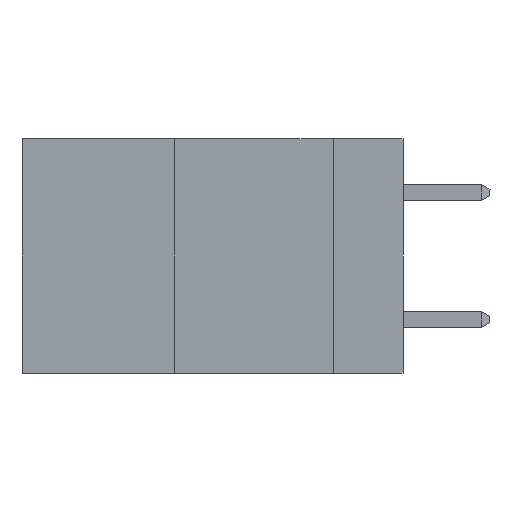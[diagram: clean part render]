
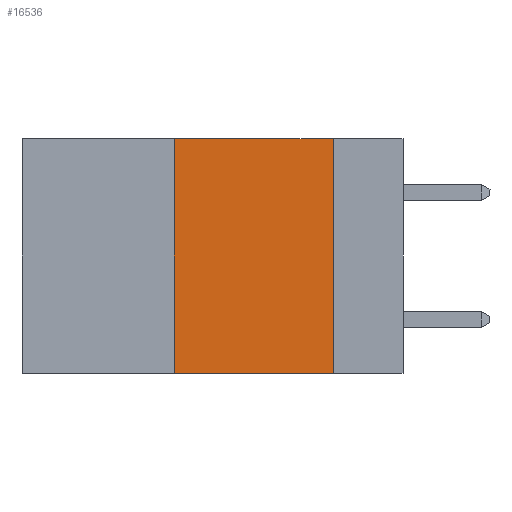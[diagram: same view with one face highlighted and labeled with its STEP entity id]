
A CAD part, left-side view. The second image highlights one B-rep face of the part: STEP entity #16536.
In plain terms, the highlighted planar face has unit normal (-1, 0, 0).
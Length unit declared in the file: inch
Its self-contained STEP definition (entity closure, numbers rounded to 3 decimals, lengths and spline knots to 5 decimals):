
#188 = EDGE_CURVE ( 'NONE', #3211, #1576, #2020, .T. ) ;
#1083 = DIRECTION ( 'NONE',  ( 0., 0., -1. ) ) ;
#1540 = VERTEX_POINT ( 'NONE', #13657 ) ;
#1576 = VERTEX_POINT ( 'NONE', #11192 ) ;
#1864 = DIRECTION ( 'NONE',  ( 1., 0., 0. ) ) ;
#2020 = LINE ( 'NONE', #2306, #15812 ) ;
#2306 = CARTESIAN_POINT ( 'NONE',  ( 0., 0.36, 0. ) ) ;
#3173 = ORIENTED_EDGE ( 'NONE', *, *, #9237, .T. ) ;
#3187 = VERTEX_POINT ( 'NONE', #14360 ) ;
#3211 = VERTEX_POINT ( 'NONE', #11871 ) ;
#3790 = EDGE_LOOP ( 'NONE', ( #7246, #5812, #7464, #3173 ) ) ;
#4678 = EDGE_CURVE ( 'NONE', #1540, #3187, #15015, .T. ) ;
#5812 = ORIENTED_EDGE ( 'NONE', *, *, #9789, .F. ) ;
#6297 = VECTOR ( 'NONE', #15700, 39.37008 ) ;
#7246 = ORIENTED_EDGE ( 'NONE', *, *, #4678, .F. ) ;
#7379 = CARTESIAN_POINT ( 'NONE',  ( 0., 0.6, 0. ) ) ;
#7464 = ORIENTED_EDGE ( 'NONE', *, *, #188, .F. ) ;
#9237 = EDGE_CURVE ( 'NONE', #3211, #3187, #9751, .T. ) ;
#9751 = LINE ( 'NONE', #13029, #6297 ) ;
#9762 = AXIS2_PLACEMENT_3D ( 'NONE', #7379, #1864, #11307 ) ;
#9789 = EDGE_CURVE ( 'NONE', #1576, #1540, #15012, .T. ) ;
#10004 = PLANE ( 'NONE',  #9762 ) ;
#11192 = CARTESIAN_POINT ( 'NONE',  ( 0., 0.36, 0. ) ) ;
#11307 = DIRECTION ( 'NONE',  ( 0., 0., -1. ) ) ;
#11545 = VECTOR ( 'NONE', #13753, 39.37008 ) ;
#11546 = VECTOR ( 'NONE', #1083, 39.37008 ) ;
#11871 = CARTESIAN_POINT ( 'NONE',  ( 0., 0.36, -0.37 ) ) ;
#12455 = CARTESIAN_POINT ( 'NONE',  ( 0., 0.6, 0. ) ) ;
#13029 = CARTESIAN_POINT ( 'NONE',  ( 0., 0.6, -0.37 ) ) ;
#13657 = CARTESIAN_POINT ( 'NONE',  ( 0., 0.11, 0. ) ) ;
#13753 = DIRECTION ( 'NONE',  ( 0., -1., 0. ) ) ;
#14233 = DIRECTION ( 'NONE',  ( 0., 0., 1. ) ) ;
#14360 = CARTESIAN_POINT ( 'NONE',  ( 0., 0.11, -0.37 ) ) ;
#14610 = FACE_OUTER_BOUND ( 'NONE', #3790, .T. ) ;
#15012 = LINE ( 'NONE', #12455, #11545 ) ;
#15015 = LINE ( 'NONE', #15815, #11546 ) ;
#15700 = DIRECTION ( 'NONE',  ( 0., -1., 0. ) ) ;
#15812 = VECTOR ( 'NONE', #14233, 39.37008 ) ;
#15815 = CARTESIAN_POINT ( 'NONE',  ( 0., 0.11, 0. ) ) ;
#16536 = ADVANCED_FACE ( 'NONE', ( #14610 ), #10004, .F. ) ;
